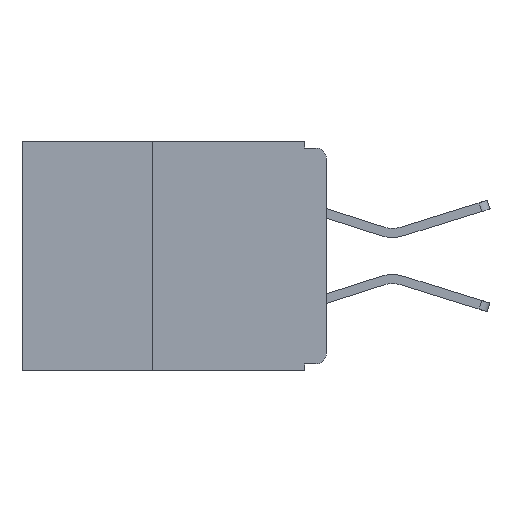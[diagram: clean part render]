
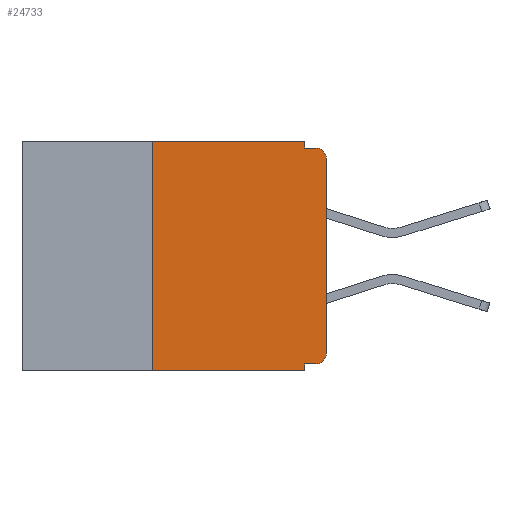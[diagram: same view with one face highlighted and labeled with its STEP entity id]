
A CAD part, left-side view. The second image highlights one B-rep face of the part: STEP entity #24733.
In plain terms, the highlighted planar face has unit normal (-1, 0, 0).
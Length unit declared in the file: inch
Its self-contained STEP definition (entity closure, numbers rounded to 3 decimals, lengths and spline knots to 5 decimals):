
#980 = ORIENTED_EDGE ( 'NONE', *, *, #13803, .F. ) ;
#996 = CARTESIAN_POINT ( 'NONE',  ( 0., 0.015, -0.32 ) ) ;
#1572 = VECTOR ( 'NONE', #14009, 39.37008 ) ;
#1619 = DIRECTION ( 'NONE',  ( 0., 0., -1. ) ) ;
#2045 = CARTESIAN_POINT ( 'NONE',  ( 0., 0., 0. ) ) ;
#2216 = EDGE_CURVE ( 'NONE', #3812, #14920, #19785, .T. ) ;
#2463 = EDGE_CURVE ( 'NONE', #4429, #6790, #25283, .T. ) ;
#2611 = CARTESIAN_POINT ( 'NONE',  ( 0., 0.031, 0. ) ) ;
#2875 = CARTESIAN_POINT ( 'NONE',  ( 0., 0.031, -0.32 ) ) ;
#3034 = CARTESIAN_POINT ( 'NONE',  ( 0., 0., -0.32 ) ) ;
#3148 = LINE ( 'NONE', #26581, #7575 ) ;
#3812 = VERTEX_POINT ( 'NONE', #19910 ) ;
#4343 = DIRECTION ( 'NONE',  ( 0., 0., -1. ) ) ;
#4350 = VERTEX_POINT ( 'NONE', #4812 ) ;
#4377 = DIRECTION ( 'NONE',  ( -1., 0., 0. ) ) ;
#4409 = CARTESIAN_POINT ( 'NONE',  ( 0., 0.015, -0.025 ) ) ;
#4429 = VERTEX_POINT ( 'NONE', #2611 ) ;
#4812 = CARTESIAN_POINT ( 'NONE',  ( 0., 0.25, -0.33 ) ) ;
#4980 = CARTESIAN_POINT ( 'NONE',  ( 0., 0., -0.01 ) ) ;
#5170 = CARTESIAN_POINT ( 'NONE',  ( 0., 0.031, -0.33 ) ) ;
#5324 = VECTOR ( 'NONE', #26520, 39.37008 ) ;
#5328 = CARTESIAN_POINT ( 'NONE',  ( 0., 0.25, -0.33 ) ) ;
#5989 = LINE ( 'NONE', #2045, #5324 ) ;
#6567 = VERTEX_POINT ( 'NONE', #20702 ) ;
#6586 = VECTOR ( 'NONE', #19677, 39.37008 ) ;
#6616 = VERTEX_POINT ( 'NONE', #19689 ) ;
#6790 = VERTEX_POINT ( 'NONE', #17389 ) ;
#6843 = ORIENTED_EDGE ( 'NONE', *, *, #26095, .F. ) ;
#7171 = DIRECTION ( 'NONE',  ( 0., -1., 0. ) ) ;
#7575 = VECTOR ( 'NONE', #20792, 39.37008 ) ;
#7632 = CARTESIAN_POINT ( 'NONE',  ( 0., 0.437, 0. ) ) ;
#9631 = EDGE_LOOP ( 'NONE', ( #22672, #16384, #980, #24202, #23904, #25139, #15137, #6843, #19984, #17761 ) ) ;
#9674 = DIRECTION ( 'NONE',  ( 0., 0., -1. ) ) ;
#9758 = AXIS2_PLACEMENT_3D ( 'NONE', #23652, #11601, #25606 ) ;
#10237 = EDGE_CURVE ( 'NONE', #10292, #26471, #18020, .T. ) ;
#10292 = VERTEX_POINT ( 'NONE', #996 ) ;
#10299 = AXIS2_PLACEMENT_3D ( 'NONE', #4409, #4377, #4343 ) ;
#11071 = CARTESIAN_POINT ( 'NONE',  ( 0., 0.015, -0.01 ) ) ;
#11601 = DIRECTION ( 'NONE',  ( -1., 0., 0. ) ) ;
#12032 = VECTOR ( 'NONE', #1619, 39.37008 ) ;
#12598 = VECTOR ( 'NONE', #17551, 39.37008 ) ;
#13103 = DIRECTION ( 'NONE',  ( 0., 0., -1. ) ) ;
#13803 = EDGE_CURVE ( 'NONE', #6790, #14920, #22246, .T. ) ;
#13918 = CARTESIAN_POINT ( 'NONE',  ( 0., 0.437, 0. ) ) ;
#14009 = DIRECTION ( 'NONE',  ( 0., -1., 0. ) ) ;
#14026 = VECTOR ( 'NONE', #13103, 39.37008 ) ;
#14920 = VERTEX_POINT ( 'NONE', #11071 ) ;
#15058 = EDGE_CURVE ( 'NONE', #4350, #6616, #17443, .T. ) ;
#15137 = ORIENTED_EDGE ( 'NONE', *, *, #26242, .T. ) ;
#16384 = ORIENTED_EDGE ( 'NONE', *, *, #2216, .T. ) ;
#17389 = CARTESIAN_POINT ( 'NONE',  ( 0., 0.031, -0.01 ) ) ;
#17443 = LINE ( 'NONE', #5328, #6586 ) ;
#17551 = DIRECTION ( 'NONE',  ( 0., 1., 0. ) ) ;
#17761 = ORIENTED_EDGE ( 'NONE', *, *, #18924, .T. ) ;
#18020 = LINE ( 'NONE', #3034, #12598 ) ;
#18210 = LINE ( 'NONE', #13918, #1572 ) ;
#18366 = EDGE_CURVE ( 'NONE', #6616, #4429, #18210, .T. ) ;
#18924 = EDGE_CURVE ( 'NONE', #10292, #6567, #20428, .T. ) ;
#19270 = EDGE_CURVE ( 'NONE', #6567, #3812, #5989, .T. ) ;
#19677 = DIRECTION ( 'NONE',  ( 0., 0., 1. ) ) ;
#19689 = CARTESIAN_POINT ( 'NONE',  ( 0., 0.25, 0. ) ) ;
#19785 = CIRCLE ( 'NONE', #10299, 0.015 ) ;
#19829 = PLANE ( 'NONE',  #24857 ) ;
#19910 = CARTESIAN_POINT ( 'NONE',  ( 0., 0., -0.025 ) ) ;
#19984 = ORIENTED_EDGE ( 'NONE', *, *, #10237, .F. ) ;
#20092 = FACE_OUTER_BOUND ( 'NONE', #9631, .T. ) ;
#20428 = CIRCLE ( 'NONE', #9758, 0.015 ) ;
#20702 = CARTESIAN_POINT ( 'NONE',  ( 0., 0., -0.305 ) ) ;
#20792 = DIRECTION ( 'NONE',  ( 0., -1., 0. ) ) ;
#21815 = DIRECTION ( 'NONE',  ( 1., 0., 0. ) ) ;
#22246 = LINE ( 'NONE', #4980, #22873 ) ;
#22672 = ORIENTED_EDGE ( 'NONE', *, *, #19270, .T. ) ;
#22783 = LINE ( 'NONE', #26176, #12032 ) ;
#22873 = VECTOR ( 'NONE', #7171, 39.37008 ) ;
#22933 = VERTEX_POINT ( 'NONE', #5170 ) ;
#23652 = CARTESIAN_POINT ( 'NONE',  ( 0., 0.015, -0.305 ) ) ;
#23904 = ORIENTED_EDGE ( 'NONE', *, *, #18366, .F. ) ;
#24202 = ORIENTED_EDGE ( 'NONE', *, *, #2463, .F. ) ;
#24733 = ADVANCED_FACE ( 'NONE', ( #20092 ), #19829, .F. ) ;
#24857 = AXIS2_PLACEMENT_3D ( 'NONE', #7632, #21815, #9674 ) ;
#25139 = ORIENTED_EDGE ( 'NONE', *, *, #15058, .F. ) ;
#25283 = LINE ( 'NONE', #26550, #14026 ) ;
#25606 = DIRECTION ( 'NONE',  ( 0., 0., -1. ) ) ;
#26095 = EDGE_CURVE ( 'NONE', #26471, #22933, #22783, .T. ) ;
#26176 = CARTESIAN_POINT ( 'NONE',  ( 0., 0.031, -0.33 ) ) ;
#26242 = EDGE_CURVE ( 'NONE', #4350, #22933, #3148, .T. ) ;
#26471 = VERTEX_POINT ( 'NONE', #2875 ) ;
#26520 = DIRECTION ( 'NONE',  ( 0., 0., 1. ) ) ;
#26550 = CARTESIAN_POINT ( 'NONE',  ( 0., 0.031, 0. ) ) ;
#26581 = CARTESIAN_POINT ( 'NONE',  ( 0., 0.437, -0.33 ) ) ;
